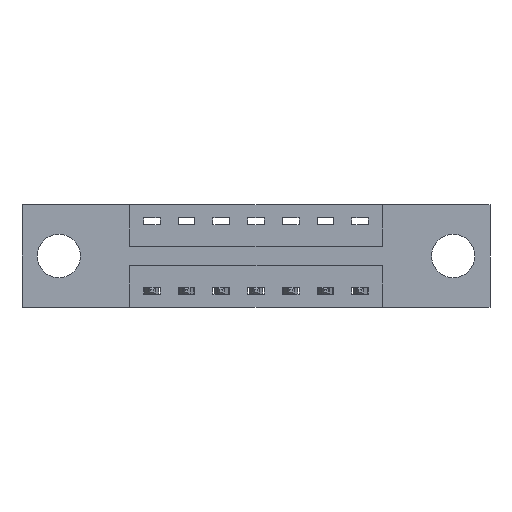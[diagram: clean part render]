
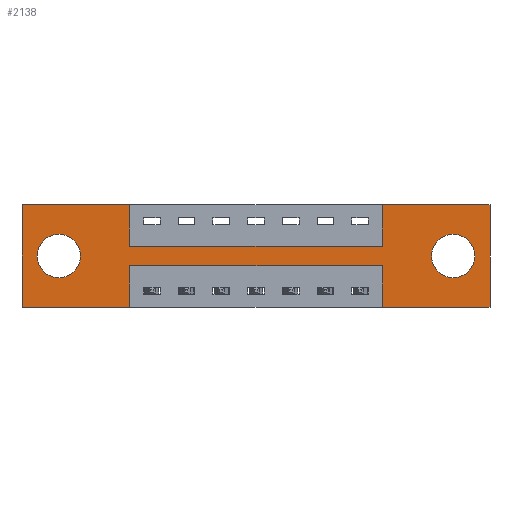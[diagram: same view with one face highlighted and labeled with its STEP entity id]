
A CAD part, front view. The second image highlights one B-rep face of the part: STEP entity #2138.
In plain terms, the highlighted planar face has unit normal (0, -1, 0).
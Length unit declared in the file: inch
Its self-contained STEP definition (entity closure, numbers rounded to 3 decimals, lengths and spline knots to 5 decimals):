
#78 = LINE ( 'NONE', #2954, #6926 ) ;
#98 = AXIS2_PLACEMENT_3D ( 'NONE', #7219, #1338, #1385 ) ;
#106 = LINE ( 'NONE', #2979, #6045 ) ;
#137 = CARTESIAN_POINT ( 'NONE',  ( 1.2975, 0., -0.37 ) ) ;
#192 = LINE ( 'NONE', #4674, #7506 ) ;
#259 = EDGE_CURVE ( 'NONE', #7311, #5727, #2188, .T. ) ;
#267 = VERTEX_POINT ( 'NONE', #8204 ) ;
#278 = CARTESIAN_POINT ( 'NONE',  ( 0.3875, 0., 0. ) ) ;
#298 = LINE ( 'NONE', #3203, #3920 ) ;
#339 = EDGE_CURVE ( 'NONE', #8652, #7664, #4480, .T. ) ;
#425 = VECTOR ( 'NONE', #6443, 39.37008 ) ;
#451 = CARTESIAN_POINT ( 'NONE',  ( 0., 0., -0.37 ) ) ;
#461 = ORIENTED_EDGE ( 'NONE', *, *, #5685, .F. ) ;
#617 = CARTESIAN_POINT ( 'NONE',  ( 0., 0., -0.37 ) ) ;
#619 = DIRECTION ( 'NONE',  ( 0., 1., 0. ) ) ;
#645 = CARTESIAN_POINT ( 'NONE',  ( 1.5525, 0., -0.185 ) ) ;
#667 = DIRECTION ( 'NONE',  ( 0., 0., -1. ) ) ;
#686 = CARTESIAN_POINT ( 'NONE',  ( 0.1325, 0., -0.263 ) ) ;
#796 = ORIENTED_EDGE ( 'NONE', *, *, #840, .F. ) ;
#840 = EDGE_CURVE ( 'NONE', #8237, #8652, #106, .T. ) ;
#885 = DIRECTION ( 'NONE',  ( 0., 0., 1. ) ) ;
#950 = CARTESIAN_POINT ( 'NONE',  ( 0., 0., 0. ) ) ;
#1288 = AXIS2_PLACEMENT_3D ( 'NONE', #645, #2114, #5924 ) ;
#1338 = DIRECTION ( 'NONE',  ( 0., 1., 0. ) ) ;
#1348 = FACE_BOUND ( 'NONE', #3531, .T. ) ;
#1368 = EDGE_CURVE ( 'NONE', #8428, #7528, #3122, .T. ) ;
#1385 = DIRECTION ( 'NONE',  ( 0., 0., -1. ) ) ;
#1403 = VERTEX_POINT ( 'NONE', #3865 ) ;
#1902 = DIRECTION ( 'NONE',  ( 0., 0., 1. ) ) ;
#2025 = ORIENTED_EDGE ( 'NONE', *, *, #5498, .T. ) ;
#2092 = DIRECTION ( 'NONE',  ( 0., 0., 1. ) ) ;
#2114 = DIRECTION ( 'NONE',  ( 0., 1., 0. ) ) ;
#2117 = DIRECTION ( 'NONE',  ( -1., 0., 0. ) ) ;
#2133 = VECTOR ( 'NONE', #2092, 39.37008 ) ;
#2138 = ADVANCED_FACE ( 'NONE', ( #1348, #3403, #4224 ), #4911, .T. ) ;
#2165 = LINE ( 'NONE', #5926, #8116 ) ;
#2188 = CIRCLE ( 'NONE', #1288, 0.078 ) ;
#2209 = DIRECTION ( 'NONE',  ( 1., 0., 0. ) ) ;
#2242 = ORIENTED_EDGE ( 'NONE', *, *, #6288, .T. ) ;
#2344 = ORIENTED_EDGE ( 'NONE', *, *, #6051, .F. ) ;
#2489 = EDGE_CURVE ( 'NONE', #5216, #7332, #298, .T. ) ;
#2624 = EDGE_CURVE ( 'NONE', #267, #1403, #4809, .T. ) ;
#2743 = EDGE_CURVE ( 'NONE', #1403, #3836, #8847, .T. ) ;
#2859 = CIRCLE ( 'NONE', #98, 0.078 ) ;
#2954 = CARTESIAN_POINT ( 'NONE',  ( 1.2975, 0., 0. ) ) ;
#2979 = CARTESIAN_POINT ( 'NONE',  ( 0., 0., 0. ) ) ;
#3122 = CIRCLE ( 'NONE', #5289, 0.078 ) ;
#3132 = ORIENTED_EDGE ( 'NONE', *, *, #259, .T. ) ;
#3198 = AXIS2_PLACEMENT_3D ( 'NONE', #8653, #619, #7044 ) ;
#3203 = CARTESIAN_POINT ( 'NONE',  ( 0., 0., 0. ) ) ;
#3403 = FACE_BOUND ( 'NONE', #4855, .T. ) ;
#3493 = CARTESIAN_POINT ( 'NONE',  ( 0.3875, 0., -0.22 ) ) ;
#3531 = EDGE_LOOP ( 'NONE', ( #2242, #3132 ) ) ;
#3549 = DIRECTION ( 'NONE',  ( 0., -1., 0. ) ) ;
#3696 = VECTOR ( 'NONE', #8564, 39.37008 ) ;
#3740 = CARTESIAN_POINT ( 'NONE',  ( 0., 0., -0.37 ) ) ;
#3836 = VERTEX_POINT ( 'NONE', #7173 ) ;
#3865 = CARTESIAN_POINT ( 'NONE',  ( 0.3875, 0., -0.22 ) ) ;
#3920 = VECTOR ( 'NONE', #6153, 39.37008 ) ;
#3921 = VERTEX_POINT ( 'NONE', #5905 ) ;
#3923 = ORIENTED_EDGE ( 'NONE', *, *, #4424, .F. ) ;
#3983 = EDGE_CURVE ( 'NONE', #8087, #267, #6690, .T. ) ;
#4046 = VECTOR ( 'NONE', #4528, 39.37008 ) ;
#4119 = DIRECTION ( 'NONE',  ( 0., 1., 0. ) ) ;
#4202 = EDGE_CURVE ( 'NONE', #3836, #8237, #5612, .T. ) ;
#4224 = FACE_OUTER_BOUND ( 'NONE', #6328, .T. ) ;
#4304 = VECTOR ( 'NONE', #5990, 39.37008 ) ;
#4391 = ORIENTED_EDGE ( 'NONE', *, *, #5848, .F. ) ;
#4424 = EDGE_CURVE ( 'NONE', #7332, #5405, #8132, .T. ) ;
#4480 = LINE ( 'NONE', #6838, #4046 ) ;
#4506 = ORIENTED_EDGE ( 'NONE', *, *, #4788, .F. ) ;
#4528 = DIRECTION ( 'NONE',  ( 1., 0., 0. ) ) ;
#4600 = CARTESIAN_POINT ( 'NONE',  ( 1.685, 0., 0. ) ) ;
#4602 = LINE ( 'NONE', #278, #7500 ) ;
#4674 = CARTESIAN_POINT ( 'NONE',  ( 0.3875, 0., -0.15 ) ) ;
#4788 = EDGE_CURVE ( 'NONE', #5405, #8087, #2165, .T. ) ;
#4809 = LINE ( 'NONE', #3493, #425 ) ;
#4824 = DIRECTION ( 'NONE',  ( 0., 0., -1. ) ) ;
#4855 = EDGE_LOOP ( 'NONE', ( #8301, #2025 ) ) ;
#4911 = PLANE ( 'NONE',  #8853 ) ;
#4952 = CARTESIAN_POINT ( 'NONE',  ( 1.2975, 0., 0. ) ) ;
#5131 = CARTESIAN_POINT ( 'NONE',  ( 0.3875, 0., -0.37 ) ) ;
#5168 = DIRECTION ( 'NONE',  ( 0., 0., 1. ) ) ;
#5216 = VERTEX_POINT ( 'NONE', #4952 ) ;
#5239 = CARTESIAN_POINT ( 'NONE',  ( 1.685, 0., 0. ) ) ;
#5289 = AXIS2_PLACEMENT_3D ( 'NONE', #5563, #4119, #1902 ) ;
#5405 = VERTEX_POINT ( 'NONE', #8240 ) ;
#5498 = EDGE_CURVE ( 'NONE', #7528, #8428, #7980, .T. ) ;
#5563 = CARTESIAN_POINT ( 'NONE',  ( 0.1325, 0., -0.185 ) ) ;
#5612 = LINE ( 'NONE', #617, #3696 ) ;
#5685 = EDGE_CURVE ( 'NONE', #7347, #5216, #78, .T. ) ;
#5727 = VERTEX_POINT ( 'NONE', #7976 ) ;
#5790 = ORIENTED_EDGE ( 'NONE', *, *, #2743, .F. ) ;
#5848 = EDGE_CURVE ( 'NONE', #7664, #3921, #4602, .T. ) ;
#5905 = CARTESIAN_POINT ( 'NONE',  ( 0.3875, 0., -0.15 ) ) ;
#5924 = DIRECTION ( 'NONE',  ( 0., 0., -1. ) ) ;
#5926 = CARTESIAN_POINT ( 'NONE',  ( 0., 0., -0.37 ) ) ;
#5990 = DIRECTION ( 'NONE',  ( 0., 0., -1. ) ) ;
#6045 = VECTOR ( 'NONE', #885, 39.37008 ) ;
#6051 = EDGE_CURVE ( 'NONE', #3921, #7347, #192, .T. ) ;
#6153 = DIRECTION ( 'NONE',  ( 1., 0., 0. ) ) ;
#6193 = ORIENTED_EDGE ( 'NONE', *, *, #339, .F. ) ;
#6288 = EDGE_CURVE ( 'NONE', #5727, #7311, #2859, .T. ) ;
#6328 = EDGE_LOOP ( 'NONE', ( #5790, #9307, #8866, #4506, #3923, #8271, #461, #2344, #4391, #6193, #796, #9078 ) ) ;
#6443 = DIRECTION ( 'NONE',  ( -1., 0., 0. ) ) ;
#6690 = LINE ( 'NONE', #137, #2133 ) ;
#6838 = CARTESIAN_POINT ( 'NONE',  ( 0., 0., 0. ) ) ;
#6926 = VECTOR ( 'NONE', #5168, 39.37008 ) ;
#6967 = CARTESIAN_POINT ( 'NONE',  ( 0.3875, 0., 0. ) ) ;
#7044 = DIRECTION ( 'NONE',  ( 0., 0., 1. ) ) ;
#7173 = CARTESIAN_POINT ( 'NONE',  ( 0.3875, 0., -0.37 ) ) ;
#7219 = CARTESIAN_POINT ( 'NONE',  ( 1.5525, 0., -0.185 ) ) ;
#7311 = VERTEX_POINT ( 'NONE', #8156 ) ;
#7332 = VERTEX_POINT ( 'NONE', #5239 ) ;
#7347 = VERTEX_POINT ( 'NONE', #8249 ) ;
#7375 = CARTESIAN_POINT ( 'NONE',  ( 1.2975, 0., -0.37 ) ) ;
#7500 = VECTOR ( 'NONE', #9118, 39.37008 ) ;
#7506 = VECTOR ( 'NONE', #2209, 39.37008 ) ;
#7528 = VERTEX_POINT ( 'NONE', #686 ) ;
#7664 = VERTEX_POINT ( 'NONE', #6967 ) ;
#7799 = VECTOR ( 'NONE', #667, 39.37008 ) ;
#7976 = CARTESIAN_POINT ( 'NONE',  ( 1.5525, 0., -0.107 ) ) ;
#7980 = CIRCLE ( 'NONE', #3198, 0.078 ) ;
#8087 = VERTEX_POINT ( 'NONE', #7375 ) ;
#8116 = VECTOR ( 'NONE', #2117, 39.37008 ) ;
#8132 = LINE ( 'NONE', #4600, #4304 ) ;
#8156 = CARTESIAN_POINT ( 'NONE',  ( 1.5525, 0., -0.263 ) ) ;
#8204 = CARTESIAN_POINT ( 'NONE',  ( 1.2975, 0., -0.22 ) ) ;
#8237 = VERTEX_POINT ( 'NONE', #3740 ) ;
#8240 = CARTESIAN_POINT ( 'NONE',  ( 1.685, 0., -0.37 ) ) ;
#8249 = CARTESIAN_POINT ( 'NONE',  ( 1.2975, 0., -0.15 ) ) ;
#8271 = ORIENTED_EDGE ( 'NONE', *, *, #2489, .F. ) ;
#8301 = ORIENTED_EDGE ( 'NONE', *, *, #1368, .T. ) ;
#8428 = VERTEX_POINT ( 'NONE', #8519 ) ;
#8519 = CARTESIAN_POINT ( 'NONE',  ( 0.1325, 0., -0.107 ) ) ;
#8564 = DIRECTION ( 'NONE',  ( -1., 0., 0. ) ) ;
#8652 = VERTEX_POINT ( 'NONE', #950 ) ;
#8653 = CARTESIAN_POINT ( 'NONE',  ( 0.1325, 0., -0.185 ) ) ;
#8847 = LINE ( 'NONE', #5131, #7799 ) ;
#8853 = AXIS2_PLACEMENT_3D ( 'NONE', #451, #3549, #4824 ) ;
#8866 = ORIENTED_EDGE ( 'NONE', *, *, #3983, .F. ) ;
#9078 = ORIENTED_EDGE ( 'NONE', *, *, #4202, .F. ) ;
#9118 = DIRECTION ( 'NONE',  ( 0., 0., -1. ) ) ;
#9307 = ORIENTED_EDGE ( 'NONE', *, *, #2624, .F. ) ;
